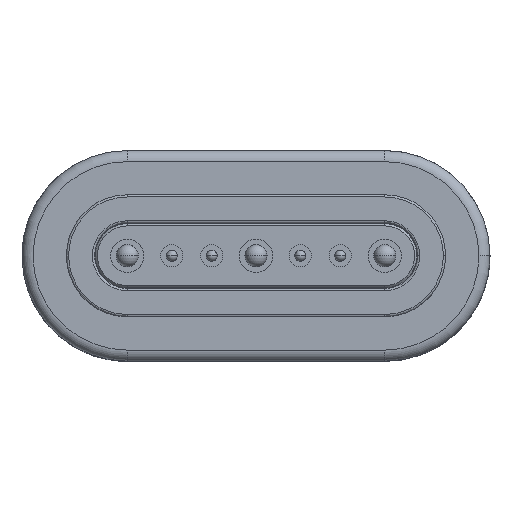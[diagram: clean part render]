
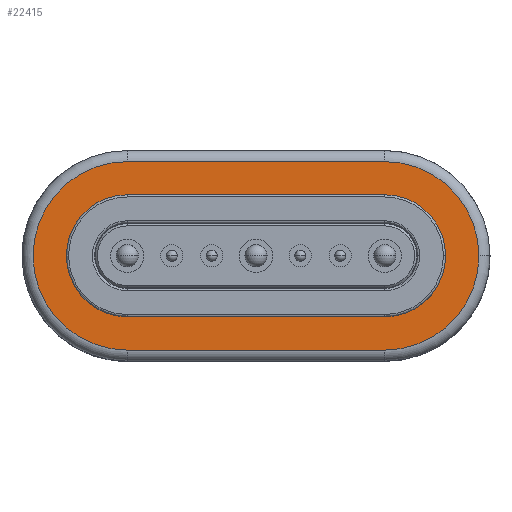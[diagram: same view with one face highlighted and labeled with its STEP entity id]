
A CAD part, top view. The second image highlights one B-rep face of the part: STEP entity #22415.
In plain terms, the highlighted planar face has unit normal (0, 0, 1).
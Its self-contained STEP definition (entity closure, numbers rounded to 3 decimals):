
#82 = AXIS2_PLACEMENT_3D ( 'NONE', #18109, #14170, #24607 ) ;
#643 = CARTESIAN_POINT ( 'NONE',  ( 5.8, 44.25, -2.8 ) ) ;
#929 = CARTESIAN_POINT ( 'NONE',  ( -5.8, 35.75, -2.8 ) ) ;
#1025 = ORIENTED_EDGE ( 'NONE', *, *, #10378, .F. ) ;
#1172 = FACE_OUTER_BOUND ( 'NONE', #16409, .T. ) ;
#1236 = ORIENTED_EDGE ( 'NONE', *, *, #19700, .T. ) ;
#1407 = VERTEX_POINT ( 'NONE', #23121 ) ;
#2331 = EDGE_CURVE ( 'NONE', #27394, #10997, #17769, .T. ) ;
#2749 = AXIS2_PLACEMENT_3D ( 'NONE', #16339, #26625, #27060 ) ;
#3002 = EDGE_CURVE ( 'NONE', #6925, #23664, #8299, .T. ) ;
#3080 = LINE ( 'NONE', #11746, #16641 ) ;
#3173 = CIRCLE ( 'NONE', #21764, 2.75 ) ;
#3401 = DIRECTION ( 'NONE',  ( 0., -1., 0. ) ) ;
#3558 = CARTESIAN_POINT ( 'NONE',  ( 5.8, 35.75, -2.8 ) ) ;
#3767 = AXIS2_PLACEMENT_3D ( 'NONE', #9969, #14334, #16319 ) ;
#4097 = VERTEX_POINT ( 'NONE', #17109 ) ;
#4208 = EDGE_LOOP ( 'NONE', ( #24108, #1236, #24444, #19746, #4940 ) ) ;
#4399 = DIRECTION ( 'NONE',  ( 0., 0., -1. ) ) ;
#4567 = CARTESIAN_POINT ( 'NONE',  ( -5.8, 37.25, -2.8 ) ) ;
#4940 = ORIENTED_EDGE ( 'NONE', *, *, #14141, .T. ) ;
#4962 = CARTESIAN_POINT ( 'NONE',  ( 5.8, 37.25, -2.8 ) ) ;
#5488 = DIRECTION ( 'NONE',  ( 0., 1., 0. ) ) ;
#5673 = CARTESIAN_POINT ( 'NONE',  ( -5.8, 40., -2.8 ) ) ;
#5938 = AXIS2_PLACEMENT_3D ( 'NONE', #12928, #4399, #8520 ) ;
#6017 = CIRCLE ( 'NONE', #3767, 4.25 ) ;
#6857 = ORIENTED_EDGE ( 'NONE', *, *, #16342, .T. ) ;
#6925 = VERTEX_POINT ( 'NONE', #4567 ) ;
#6935 = AXIS2_PLACEMENT_3D ( 'NONE', #5673, #14183, #3401 ) ;
#7566 = CARTESIAN_POINT ( 'NONE',  ( -5.8, 37.25, -2.8 ) ) ;
#7688 = DIRECTION ( 'NONE',  ( 0., 1., 0. ) ) ;
#8243 = VECTOR ( 'NONE', #11708, 1000. ) ;
#8299 = CIRCLE ( 'NONE', #6935, 2.75 ) ;
#8364 = ORIENTED_EDGE ( 'NONE', *, *, #2331, .T. ) ;
#8520 = DIRECTION ( 'NONE',  ( 0., -1., 0. ) ) ;
#9969 = CARTESIAN_POINT ( 'NONE',  ( 5.8, 40., -2.8 ) ) ;
#10057 = CIRCLE ( 'NONE', #82, 2.75 ) ;
#10329 = VERTEX_POINT ( 'NONE', #4962 ) ;
#10378 = EDGE_CURVE ( 'NONE', #4097, #24694, #15169, .T. ) ;
#10520 = CARTESIAN_POINT ( 'NONE',  ( -8.55, 40., -2.8 ) ) ;
#10997 = VERTEX_POINT ( 'NONE', #15464 ) ;
#11629 = VERTEX_POINT ( 'NONE', #26612 ) ;
#11708 = DIRECTION ( 'NONE',  ( 1., 0., 0. ) ) ;
#11746 = CARTESIAN_POINT ( 'NONE',  ( 5.8, 42.75, -2.8 ) ) ;
#12130 = FACE_BOUND ( 'NONE', #4208, .T. ) ;
#12775 = CARTESIAN_POINT ( 'NONE',  ( -5.8, 35.75, -2.8 ) ) ;
#12838 = CARTESIAN_POINT ( 'NONE',  ( 5.8, 40., -2.8 ) ) ;
#12928 = CARTESIAN_POINT ( 'NONE',  ( -5.8, 40., -2.8 ) ) ;
#13939 = EDGE_CURVE ( 'NONE', #27022, #10997, #14534, .T. ) ;
#14141 = EDGE_CURVE ( 'NONE', #23664, #11629, #10057, .T. ) ;
#14170 = DIRECTION ( 'NONE',  ( 0., 0., -1. ) ) ;
#14183 = DIRECTION ( 'NONE',  ( 0., 0., -1. ) ) ;
#14224 = PLANE ( 'NONE',  #2749 ) ;
#14334 = DIRECTION ( 'NONE',  ( 0., 0., -1. ) ) ;
#14534 = CIRCLE ( 'NONE', #5938, 4.25 ) ;
#15169 = CIRCLE ( 'NONE', #18317, 4.25 ) ;
#15464 = CARTESIAN_POINT ( 'NONE',  ( -5.8, 44.25, -2.8 ) ) ;
#16121 = DIRECTION ( 'NONE',  ( -1., 0., 0. ) ) ;
#16319 = DIRECTION ( 'NONE',  ( 0., 1., 0. ) ) ;
#16339 = CARTESIAN_POINT ( 'NONE',  ( 0., 40., -2.8 ) ) ;
#16342 = EDGE_CURVE ( 'NONE', #27022, #24694, #20938, .T. ) ;
#16409 = EDGE_LOOP ( 'NONE', ( #24482, #8364, #26172, #6857, #1025 ) ) ;
#16641 = VECTOR ( 'NONE', #16121, 1000. ) ;
#16854 = VECTOR ( 'NONE', #26239, 1000. ) ;
#17109 = CARTESIAN_POINT ( 'NONE',  ( 10.05, 40., -2.8 ) ) ;
#17769 = LINE ( 'NONE', #643, #16854 ) ;
#18109 = CARTESIAN_POINT ( 'NONE',  ( -5.8, 40., -2.8 ) ) ;
#18317 = AXIS2_PLACEMENT_3D ( 'NONE', #20209, #20335, #5488 ) ;
#19700 = EDGE_CURVE ( 'NONE', #1407, #10329, #3173, .T. ) ;
#19746 = ORIENTED_EDGE ( 'NONE', *, *, #3002, .T. ) ;
#20209 = CARTESIAN_POINT ( 'NONE',  ( 5.8, 40., -2.8 ) ) ;
#20335 = DIRECTION ( 'NONE',  ( 0., 0., -1. ) ) ;
#20578 = LINE ( 'NONE', #7566, #8243 ) ;
#20641 = EDGE_CURVE ( 'NONE', #6925, #10329, #20578, .T. ) ;
#20938 = LINE ( 'NONE', #12775, #21559 ) ;
#21559 = VECTOR ( 'NONE', #27715, 1000. ) ;
#21764 = AXIS2_PLACEMENT_3D ( 'NONE', #12838, #26479, #7688 ) ;
#22415 = ADVANCED_FACE ( 'NONE', ( #1172, #12130 ), #14224, .T. ) ;
#23121 = CARTESIAN_POINT ( 'NONE',  ( 5.8, 42.75, -2.8 ) ) ;
#23664 = VERTEX_POINT ( 'NONE', #10520 ) ;
#24108 = ORIENTED_EDGE ( 'NONE', *, *, #27021, .F. ) ;
#24444 = ORIENTED_EDGE ( 'NONE', *, *, #20641, .F. ) ;
#24482 = ORIENTED_EDGE ( 'NONE', *, *, #24665, .F. ) ;
#24607 = DIRECTION ( 'NONE',  ( 0., -1., 0. ) ) ;
#24665 = EDGE_CURVE ( 'NONE', #27394, #4097, #6017, .T. ) ;
#24694 = VERTEX_POINT ( 'NONE', #3558 ) ;
#26172 = ORIENTED_EDGE ( 'NONE', *, *, #13939, .F. ) ;
#26239 = DIRECTION ( 'NONE',  ( -1., 0., 0. ) ) ;
#26479 = DIRECTION ( 'NONE',  ( 0., 0., -1. ) ) ;
#26612 = CARTESIAN_POINT ( 'NONE',  ( -5.8, 42.75, -2.8 ) ) ;
#26625 = DIRECTION ( 'NONE',  ( 0., 0., 1. ) ) ;
#27021 = EDGE_CURVE ( 'NONE', #1407, #11629, #3080, .T. ) ;
#27022 = VERTEX_POINT ( 'NONE', #929 ) ;
#27060 = DIRECTION ( 'NONE',  ( 1., 0., 0. ) ) ;
#27063 = CARTESIAN_POINT ( 'NONE',  ( 5.8, 44.25, -2.8 ) ) ;
#27394 = VERTEX_POINT ( 'NONE', #27063 ) ;
#27715 = DIRECTION ( 'NONE',  ( 1., 0., 0. ) ) ;
